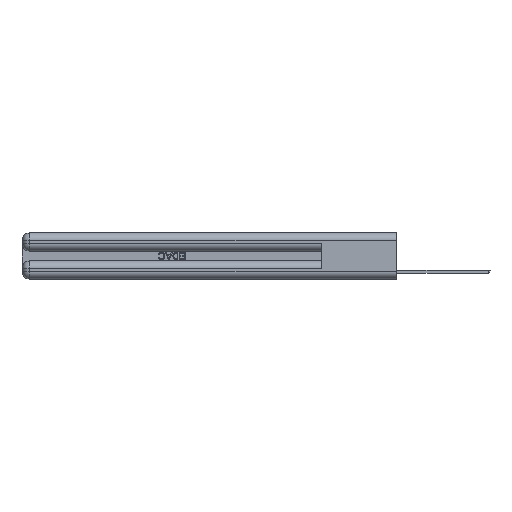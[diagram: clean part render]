
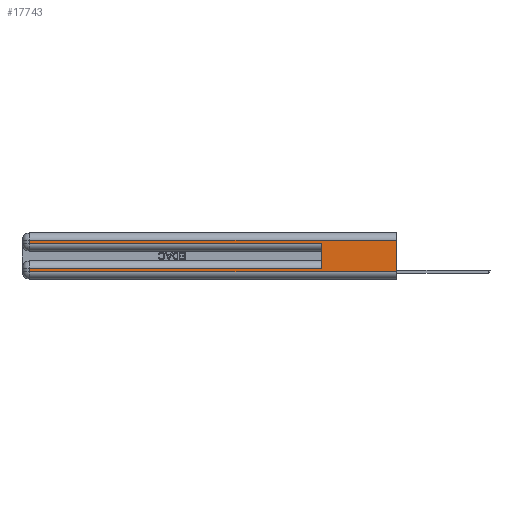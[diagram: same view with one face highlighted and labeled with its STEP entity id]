
A CAD part, left-side view. The second image highlights one B-rep face of the part: STEP entity #17743.
In plain terms, the highlighted planar face has unit normal (-1, 0, 0).
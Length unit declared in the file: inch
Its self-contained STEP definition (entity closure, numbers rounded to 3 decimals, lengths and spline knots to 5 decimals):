
#1088 = LINE ( 'NONE', #32231, #9939 ) ;
#2233 = CARTESIAN_POINT ( 'NONE',  ( 0., 0., 0.37 ) ) ;
#2334 = DIRECTION ( 'NONE',  ( 0., -1., 0. ) ) ;
#2468 = VERTEX_POINT ( 'NONE', #15281 ) ;
#2826 = CARTESIAN_POINT ( 'NONE',  ( 0., 2.94, 0.31 ) ) ;
#3007 = DIRECTION ( 'NONE',  ( 0., 1., 0. ) ) ;
#3503 = EDGE_CURVE ( 'NONE', #2468, #13150, #1088, .T. ) ;
#4404 = VERTEX_POINT ( 'NONE', #30722 ) ;
#4434 = ORIENTED_EDGE ( 'NONE', *, *, #20951, .T. ) ;
#5248 = ORIENTED_EDGE ( 'NONE', *, *, #3503, .T. ) ;
#5318 = CARTESIAN_POINT ( 'NONE',  ( 0., 2.94, 0.37 ) ) ;
#5405 = CARTESIAN_POINT ( 'NONE',  ( 0., 2.94, 0.085 ) ) ;
#5721 = VECTOR ( 'NONE', #26280, 39.37008 ) ;
#6072 = CARTESIAN_POINT ( 'NONE',  ( 0., 0., 0.31 ) ) ;
#6661 = ORIENTED_EDGE ( 'NONE', *, *, #30437, .T. ) ;
#6734 = VERTEX_POINT ( 'NONE', #31968 ) ;
#7267 = CARTESIAN_POINT ( 'NONE',  ( 0., 0., 0.31 ) ) ;
#7315 = VECTOR ( 'NONE', #26408, 39.37008 ) ;
#7363 = CARTESIAN_POINT ( 'NONE',  ( 0., 2.94, 0.37 ) ) ;
#7389 = LINE ( 'NONE', #20683, #30196 ) ;
#8011 = ORIENTED_EDGE ( 'NONE', *, *, #17162, .T. ) ;
#8635 = CARTESIAN_POINT ( 'NONE',  ( 0., 0., 0.06 ) ) ;
#9618 = AXIS2_PLACEMENT_3D ( 'NONE', #2233, #12576, #20624 ) ;
#9702 = VECTOR ( 'NONE', #18094, 39.37008 ) ;
#9939 = VECTOR ( 'NONE', #16731, 39.37008 ) ;
#9946 = VECTOR ( 'NONE', #2334, 39.37008 ) ;
#9986 = LINE ( 'NONE', #12841, #9946 ) ;
#11645 = CARTESIAN_POINT ( 'NONE',  ( 0., 0., 0.37 ) ) ;
#12576 = DIRECTION ( 'NONE',  ( 1., 0., 0. ) ) ;
#12841 = CARTESIAN_POINT ( 'NONE',  ( 0., 0., 0.285 ) ) ;
#13150 = VERTEX_POINT ( 'NONE', #8635 ) ;
#14574 = VERTEX_POINT ( 'NONE', #2826 ) ;
#15137 = FACE_OUTER_BOUND ( 'NONE', #24380, .T. ) ;
#15281 = CARTESIAN_POINT ( 'NONE',  ( 0., 2.94, 0.06 ) ) ;
#15667 = ORIENTED_EDGE ( 'NONE', *, *, #20928, .T. ) ;
#16731 = DIRECTION ( 'NONE',  ( 0., -1., 0. ) ) ;
#17162 = EDGE_CURVE ( 'NONE', #14574, #6734, #25917, .T. ) ;
#17743 = ADVANCED_FACE ( 'NONE', ( #15137 ), #25561, .F. ) ;
#18094 = DIRECTION ( 'NONE',  ( 0., 0., -1. ) ) ;
#18830 = LINE ( 'NONE', #11645, #25864 ) ;
#20624 = DIRECTION ( 'NONE',  ( 0., 0., -1. ) ) ;
#20629 = EDGE_CURVE ( 'NONE', #21563, #13150, #18830, .T. ) ;
#20683 = CARTESIAN_POINT ( 'NONE',  ( 0., 0., 0.085 ) ) ;
#20843 = DIRECTION ( 'NONE',  ( 0., 1., 0. ) ) ;
#20928 = EDGE_CURVE ( 'NONE', #25709, #2468, #28828, .T. ) ;
#20951 = EDGE_CURVE ( 'NONE', #4404, #25709, #7389, .T. ) ;
#21475 = VERTEX_POINT ( 'NONE', #32156 ) ;
#21563 = VERTEX_POINT ( 'NONE', #7267 ) ;
#23030 = ORIENTED_EDGE ( 'NONE', *, *, #20629, .F. ) ;
#24173 = ORIENTED_EDGE ( 'NONE', *, *, #26097, .T. ) ;
#24274 = DIRECTION ( 'NONE',  ( 0., 0., -1. ) ) ;
#24380 = EDGE_LOOP ( 'NONE', ( #23030, #6661, #8011, #24173, #27525, #4434, #15667, #5248 ) ) ;
#25561 = PLANE ( 'NONE',  #9618 ) ;
#25709 = VERTEX_POINT ( 'NONE', #5405 ) ;
#25864 = VECTOR ( 'NONE', #24274, 39.37008 ) ;
#25909 = LINE ( 'NONE', #31178, #7315 ) ;
#25917 = LINE ( 'NONE', #7363, #9702 ) ;
#26097 = EDGE_CURVE ( 'NONE', #6734, #21475, #9986, .T. ) ;
#26280 = DIRECTION ( 'NONE',  ( 0., 0., -1. ) ) ;
#26408 = DIRECTION ( 'NONE',  ( 0., 0., 1. ) ) ;
#27525 = ORIENTED_EDGE ( 'NONE', *, *, #28177, .F. ) ;
#28177 = EDGE_CURVE ( 'NONE', #4404, #21475, #25909, .T. ) ;
#28828 = LINE ( 'NONE', #5318, #5721 ) ;
#29235 = LINE ( 'NONE', #6072, #29638 ) ;
#29638 = VECTOR ( 'NONE', #3007, 39.37008 ) ;
#30196 = VECTOR ( 'NONE', #20843, 39.37008 ) ;
#30437 = EDGE_CURVE ( 'NONE', #21563, #14574, #29235, .T. ) ;
#30722 = CARTESIAN_POINT ( 'NONE',  ( 0., 0.6, 0.085 ) ) ;
#31178 = CARTESIAN_POINT ( 'NONE',  ( 0., 0.6, 0.145 ) ) ;
#31968 = CARTESIAN_POINT ( 'NONE',  ( 0., 2.94, 0.285 ) ) ;
#32156 = CARTESIAN_POINT ( 'NONE',  ( 0., 0.6, 0.285 ) ) ;
#32231 = CARTESIAN_POINT ( 'NONE',  ( 0., 0., 0.06 ) ) ;
